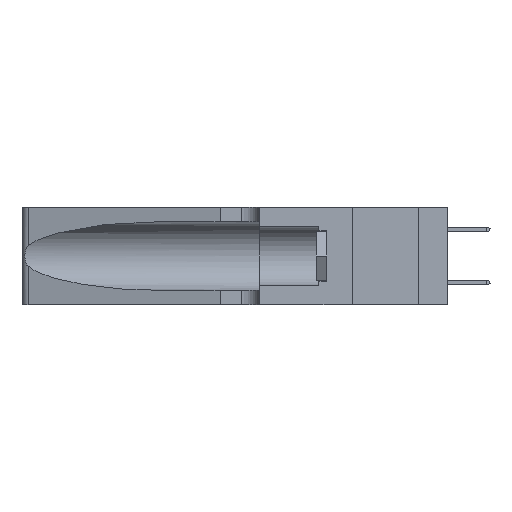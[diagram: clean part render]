
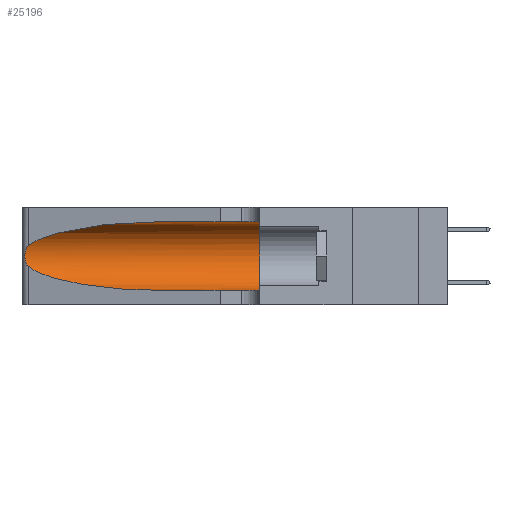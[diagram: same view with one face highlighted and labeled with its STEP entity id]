
A CAD part, left-side view. The second image highlights one B-rep face of the part: STEP entity #25196.
In plain terms, the highlighted cylindrical face has radius 3.308 mm (diameter 6.617 mm), a partial arc.
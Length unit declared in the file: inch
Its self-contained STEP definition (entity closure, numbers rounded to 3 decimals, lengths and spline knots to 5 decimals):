
#560 = CARTESIAN_POINT ( 'NONE',  ( 0.1305, 0.35, 0.185 ) ) ;
#655 = VERTEX_POINT ( 'NONE', #1061 ) ;
#670 = CARTESIAN_POINT ( 'NONE',  ( 0.25854, 1.2359, 0.20912 ) ) ;
#678 = VERTEX_POINT ( 'NONE', #1149 ) ;
#686 = LINE ( 'NONE', #2716, #12487 ) ;
#933 = DIRECTION ( 'NONE',  ( 0., -1., 0. ) ) ;
#1061 = CARTESIAN_POINT ( 'NONE',  ( 0.25487, 1.22718, 0.14631 ) ) ;
#1149 = CARTESIAN_POINT ( 'NONE',  ( 0.1305, 0.72297, 0.31525 ) ) ;
#1781 = CIRCLE ( 'NONE', #24774, 0.13025 ) ;
#2364 = EDGE_CURVE ( 'NONE', #2676, #12382, #686, .T. ) ;
#2676 = VERTEX_POINT ( 'NONE', #10764 ) ;
#2716 = CARTESIAN_POINT ( 'NONE',  ( 0.1305, 1.61858, 0.05475 ) ) ;
#2953 = DIRECTION ( 'NONE',  ( 0., 0., 1. ) ) ;
#3061 = CARTESIAN_POINT ( 'NONE',  ( 0.26075, 1.23896, 0.19203 ) ) ;
#3495 = CARTESIAN_POINT ( 'NONE',  ( 0.18966, 0.96281, 0.31525 ) ) ;
#3605 = CARTESIAN_POINT ( 'NONE',  ( 0.25487, 1.22718, 0.22369 ) ) ;
#3632 = ORIENTED_EDGE ( 'NONE', *, *, #2364, .T. ) ;
#3641 = ORIENTED_EDGE ( 'NONE', *, *, #29322, .T. ) ;
#5091 = CARTESIAN_POINT ( 'NONE',  ( 0.25487, 1.22718, 0.14631 ) ) ;
#5143 = CARTESIAN_POINT ( 'NONE',  ( 0.1305, 0.35, 0.05475 ) ) ;
#5295 = EDGE_LOOP ( 'NONE', ( #28842, #17235, #3641, #3632, #29994, #10393 ) ) ;
#5452 = CARTESIAN_POINT ( 'NONE',  ( 0.26017, 1.23833, 0.17102 ) ) ;
#6000 = VERTEX_POINT ( 'NONE', #23958 ) ;
#7026 = B_SPLINE_CURVE_WITH_KNOTS ( 'NONE', 3,
 ( #16768, #26267, #28561, #14755, #670, #17070, #3061, #19367, #5452, #21693, #8229, #24418, #10581, #26763 ),
 .UNSPECIFIED., .F., .F.,
 ( 4, 2, 2, 2, 2, 2, 4 ),
 ( 0., 0.00027, 0.00053, 0.00107, 0.0016, 0.00187, 0.00214 ),
 .UNSPECIFIED. ) ;
#8229 = CARTESIAN_POINT ( 'NONE',  ( 0.25789, 1.23486, 0.15765 ) ) ;
#8869 = VECTOR ( 'NONE', #15731, 39.37008 ) ;
#9807 = CARTESIAN_POINT ( 'NONE',  ( 0.1305, 0.72297, 0.05475 ) ) ;
#10393 = ORIENTED_EDGE ( 'NONE', *, *, #29085, .F. ) ;
#10581 = CARTESIAN_POINT ( 'NONE',  ( 0.25555, 1.22993, 0.14849 ) ) ;
#10764 = CARTESIAN_POINT ( 'NONE',  ( 0.1305, 0.72297, 0.05475 ) ) ;
#11226 =( BOUNDED_CURVE ( )  B_SPLINE_CURVE ( 3, ( #5091, #21325, #23650, #9807 ),
 .UNSPECIFIED., .F., .F. ) 
 B_SPLINE_CURVE_WITH_KNOTS ( ( 4, 4 ),
 ( 3.44316, 4.71239 ),
 .UNSPECIFIED. ) 
 CURVE ( )  GEOMETRIC_REPRESENTATION_ITEM ( )  RATIONAL_B_SPLINE_CURVE ( ( 1., 0.87, 0.87, 1. ) ) 
 REPRESENTATION_ITEM ( '' )  );
#12049 = EDGE_CURVE ( 'NONE', #678, #6000, #28085, .T. ) ;
#12382 = VERTEX_POINT ( 'NONE', #5143 ) ;
#12487 = VECTOR ( 'NONE', #14445, 39.37008 ) ;
#14125 = VERTEX_POINT ( 'NONE', #24994 ) ;
#14175 = CYLINDRICAL_SURFACE ( 'NONE', #23543, 0.13025 ) ;
#14445 = DIRECTION ( 'NONE',  ( 0., -1., 0. ) ) ;
#14755 = CARTESIAN_POINT ( 'NONE',  ( 0.25787, 1.23484, 0.2124 ) ) ;
#15037 = DIRECTION ( 'NONE',  ( 0., 0., -1. ) ) ;
#15097 = LINE ( 'NONE', #24872, #8869 ) ;
#15276 = CARTESIAN_POINT ( 'NONE',  ( 0.1305, 0.72297, 0.31525 ) ) ;
#15731 = DIRECTION ( 'NONE',  ( 0., -1., 0. ) ) ;
#16768 = CARTESIAN_POINT ( 'NONE',  ( 0.25487, 1.22718, 0.22369 ) ) ;
#16975 = DIRECTION ( 'NONE',  ( 0., 1., 0. ) ) ;
#17070 = CARTESIAN_POINT ( 'NONE',  ( 0.26018, 1.23835, 0.19895 ) ) ;
#17235 = ORIENTED_EDGE ( 'NONE', *, *, #28239, .T. ) ;
#17576 = CARTESIAN_POINT ( 'NONE',  ( 0.2373, 1.15595, 0.28018 ) ) ;
#19367 = CARTESIAN_POINT ( 'NONE',  ( 0.26075, 1.23896, 0.178 ) ) ;
#21325 = CARTESIAN_POINT ( 'NONE',  ( 0.2373, 1.15595, 0.08982 ) ) ;
#21693 = CARTESIAN_POINT ( 'NONE',  ( 0.25856, 1.23593, 0.16098 ) ) ;
#23543 = AXIS2_PLACEMENT_3D ( 'NONE', #28722, #933, #15037 ) ;
#23650 = CARTESIAN_POINT ( 'NONE',  ( 0.18966, 0.96281, 0.05475 ) ) ;
#23958 = CARTESIAN_POINT ( 'NONE',  ( 0.25487, 1.22718, 0.22369 ) ) ;
#24418 = CARTESIAN_POINT ( 'NONE',  ( 0.25639, 1.23186, 0.15144 ) ) ;
#24774 = AXIS2_PLACEMENT_3D ( 'NONE', #560, #16975, #2953 ) ;
#24872 = CARTESIAN_POINT ( 'NONE',  ( 0.1305, 1.61858, 0.31525 ) ) ;
#24994 = CARTESIAN_POINT ( 'NONE',  ( 0.1305, 0.35, 0.31525 ) ) ;
#25196 = ADVANCED_FACE ( 'NONE', ( #26479 ), #14175, .F. ) ;
#26267 = CARTESIAN_POINT ( 'NONE',  ( 0.25555, 1.22994, 0.2215 ) ) ;
#26479 = FACE_OUTER_BOUND ( 'NONE', #5295, .T. ) ;
#26763 = CARTESIAN_POINT ( 'NONE',  ( 0.25487, 1.22718, 0.14631 ) ) ;
#28085 =( BOUNDED_CURVE ( )  B_SPLINE_CURVE ( 3, ( #15276, #3495, #17576, #3605 ),
 .UNSPECIFIED., .F., .F. ) 
 B_SPLINE_CURVE_WITH_KNOTS ( ( 4, 4 ),
 ( 1.5708, 2.84003 ),
 .UNSPECIFIED. ) 
 CURVE ( )  GEOMETRIC_REPRESENTATION_ITEM ( )  RATIONAL_B_SPLINE_CURVE ( ( 1., 0.87, 0.87, 1. ) ) 
 REPRESENTATION_ITEM ( '' )  );
#28239 = EDGE_CURVE ( 'NONE', #6000, #655, #7026, .T. ) ;
#28561 = CARTESIAN_POINT ( 'NONE',  ( 0.25639, 1.23184, 0.21858 ) ) ;
#28722 = CARTESIAN_POINT ( 'NONE',  ( 0.1305, 1.61858, 0.185 ) ) ;
#28842 = ORIENTED_EDGE ( 'NONE', *, *, #12049, .T. ) ;
#29085 = EDGE_CURVE ( 'NONE', #678, #14125, #15097, .T. ) ;
#29322 = EDGE_CURVE ( 'NONE', #655, #2676, #11226, .T. ) ;
#29994 = ORIENTED_EDGE ( 'NONE', *, *, #30012, .F. ) ;
#30012 = EDGE_CURVE ( 'NONE', #14125, #12382, #1781, .T. ) ;
